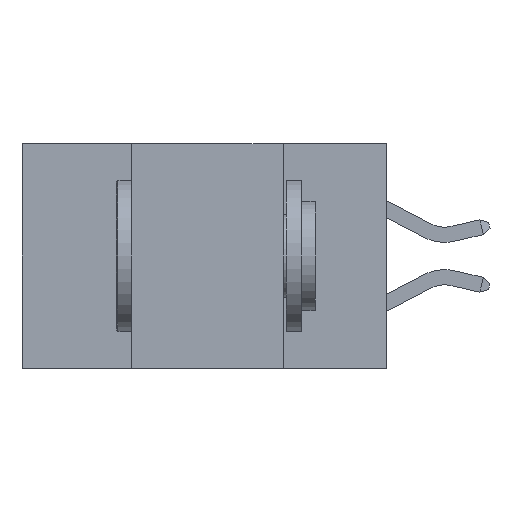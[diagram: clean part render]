
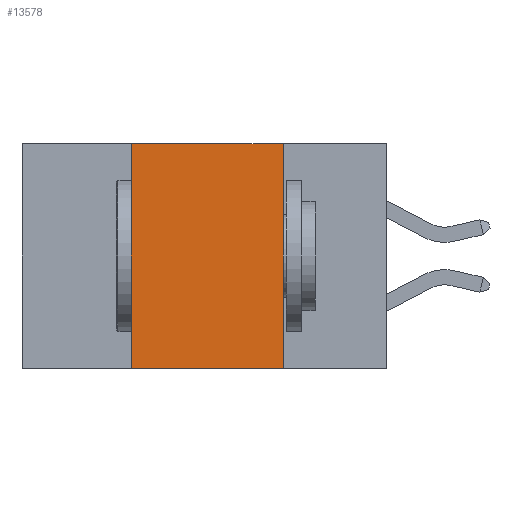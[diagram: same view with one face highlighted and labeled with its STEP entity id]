
A CAD part, left-side view. The second image highlights one B-rep face of the part: STEP entity #13578.
In plain terms, the highlighted planar face has unit normal (-1, 0, 0).
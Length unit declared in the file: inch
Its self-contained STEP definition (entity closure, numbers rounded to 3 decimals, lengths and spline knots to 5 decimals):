
#391 = VERTEX_POINT ( 'NONE', #18311 ) ;
#2043 = VECTOR ( 'NONE', #8957, 39.37008 ) ;
#2320 = ORIENTED_EDGE ( 'NONE', *, *, #18273, .F. ) ;
#2338 = VERTEX_POINT ( 'NONE', #21033 ) ;
#2693 = LINE ( 'NONE', #25642, #2043 ) ;
#2801 = AXIS2_PLACEMENT_3D ( 'NONE', #21891, #11402, #25989 ) ;
#3078 = CARTESIAN_POINT ( 'NONE',  ( 0., 0.42, 0. ) ) ;
#6036 = DIRECTION ( 'NONE',  ( 0., -1., 0. ) ) ;
#7681 = EDGE_LOOP ( 'NONE', ( #2320, #13494, #20487, #25928 ) ) ;
#7987 = CARTESIAN_POINT ( 'NONE',  ( 0., 0.17, 0. ) ) ;
#8022 = CARTESIAN_POINT ( 'NONE',  ( 0., 0.42, 0. ) ) ;
#8103 = EDGE_CURVE ( 'NONE', #2338, #391, #8204, .T. ) ;
#8204 = LINE ( 'NONE', #12267, #24215 ) ;
#8226 = CARTESIAN_POINT ( 'NONE',  ( 0., 0.17, 0. ) ) ;
#8614 = VECTOR ( 'NONE', #16454, 39.37008 ) ;
#8957 = DIRECTION ( 'NONE',  ( 0., -1., 0. ) ) ;
#10736 = LINE ( 'NONE', #8226, #21277 ) ;
#11402 = DIRECTION ( 'NONE',  ( 1., 0., 0. ) ) ;
#12267 = CARTESIAN_POINT ( 'NONE',  ( 0., 0.6, -0.37 ) ) ;
#12383 = DIRECTION ( 'NONE',  ( 0., 0., -1. ) ) ;
#13494 = ORIENTED_EDGE ( 'NONE', *, *, #19909, .F. ) ;
#13578 = ADVANCED_FACE ( 'NONE', ( #25594 ), #23932, .F. ) ;
#16454 = DIRECTION ( 'NONE',  ( 0., 0., 1. ) ) ;
#18273 = EDGE_CURVE ( 'NONE', #23380, #391, #10736, .T. ) ;
#18311 = CARTESIAN_POINT ( 'NONE',  ( 0., 0.17, -0.37 ) ) ;
#19789 = LINE ( 'NONE', #8022, #8614 ) ;
#19909 = EDGE_CURVE ( 'NONE', #23510, #23380, #2693, .T. ) ;
#20487 = ORIENTED_EDGE ( 'NONE', *, *, #26902, .F. ) ;
#21033 = CARTESIAN_POINT ( 'NONE',  ( 0., 0.42, -0.37 ) ) ;
#21277 = VECTOR ( 'NONE', #12383, 39.37008 ) ;
#21891 = CARTESIAN_POINT ( 'NONE',  ( 0., 0.6, 0. ) ) ;
#23380 = VERTEX_POINT ( 'NONE', #7987 ) ;
#23510 = VERTEX_POINT ( 'NONE', #3078 ) ;
#23932 = PLANE ( 'NONE',  #2801 ) ;
#24215 = VECTOR ( 'NONE', #6036, 39.37008 ) ;
#25594 = FACE_OUTER_BOUND ( 'NONE', #7681, .T. ) ;
#25642 = CARTESIAN_POINT ( 'NONE',  ( 0., 0.6, 0. ) ) ;
#25928 = ORIENTED_EDGE ( 'NONE', *, *, #8103, .T. ) ;
#25989 = DIRECTION ( 'NONE',  ( 0., 0., -1. ) ) ;
#26902 = EDGE_CURVE ( 'NONE', #2338, #23510, #19789, .T. ) ;
